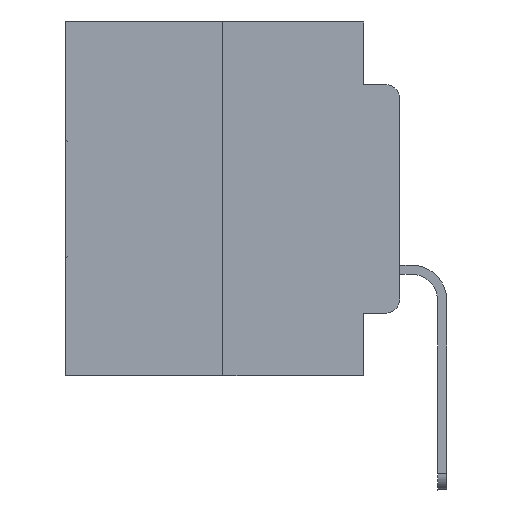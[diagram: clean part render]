
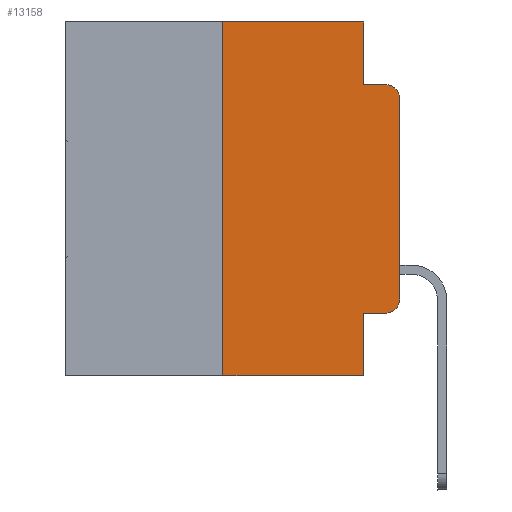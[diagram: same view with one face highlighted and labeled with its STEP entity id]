
A CAD part, left-side view. The second image highlights one B-rep face of the part: STEP entity #13158.
In plain terms, the highlighted planar face has unit normal (-1, 0, 0).
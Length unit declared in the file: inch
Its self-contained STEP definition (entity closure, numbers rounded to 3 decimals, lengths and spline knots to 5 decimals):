
#380 = LINE ( 'NONE', #9405, #19714 ) ;
#492 = DIRECTION ( 'NONE',  ( 0., 0., -1. ) ) ;
#578 = FACE_OUTER_BOUND ( 'NONE', #15499, .T. ) ;
#587 = ORIENTED_EDGE ( 'NONE', *, *, #24625, .T. ) ;
#1168 = PLANE ( 'NONE',  #5610 ) ;
#1200 = AXIS2_PLACEMENT_3D ( 'NONE', #18054, #7723, #14354 ) ;
#1474 = LINE ( 'NONE', #10653, #11525 ) ;
#1544 = CARTESIAN_POINT ( 'NONE',  ( 0., 0.02, -0.3915 ) ) ;
#1706 = VECTOR ( 'NONE', #13586, 39.37008 ) ;
#2257 = ORIENTED_EDGE ( 'NONE', *, *, #26049, .F. ) ;
#2346 = CARTESIAN_POINT ( 'NONE',  ( 0., 0.051, -0.4115 ) ) ;
#2530 = EDGE_CURVE ( 'NONE', #24203, #27634, #28332, .T. ) ;
#3697 = CIRCLE ( 'NONE', #15929, 0.02 ) ;
#4872 = CARTESIAN_POINT ( 'NONE',  ( 0., 0., 0. ) ) ;
#5607 = DIRECTION ( 'NONE',  ( 1., 0., 0. ) ) ;
#5610 = AXIS2_PLACEMENT_3D ( 'NONE', #27601, #5607, #7378 ) ;
#6230 = VERTEX_POINT ( 'NONE', #17805 ) ;
#6759 = DIRECTION ( 'NONE',  ( 0., -1., 0. ) ) ;
#7185 = DIRECTION ( 'NONE',  ( 0., 0., 1. ) ) ;
#7378 = DIRECTION ( 'NONE',  ( 0., 0., -1. ) ) ;
#7431 = CARTESIAN_POINT ( 'NONE',  ( 0., 0.051, 0. ) ) ;
#7723 = DIRECTION ( 'NONE',  ( -1., 0., 0. ) ) ;
#7748 = CARTESIAN_POINT ( 'NONE',  ( 0., 0., -0.1085 ) ) ;
#7784 = ORIENTED_EDGE ( 'NONE', *, *, #9140, .F. ) ;
#8297 = LINE ( 'NONE', #17011, #24877 ) ;
#9023 = CARTESIAN_POINT ( 'NONE',  ( 0., 0.25, 0. ) ) ;
#9140 = EDGE_CURVE ( 'NONE', #15841, #12263, #27657, .T. ) ;
#9329 = DIRECTION ( 'NONE',  ( 0., 0., -1. ) ) ;
#9405 = CARTESIAN_POINT ( 'NONE',  ( 0., 0.25, 0. ) ) ;
#10653 = CARTESIAN_POINT ( 'NONE',  ( 0., 0.051, -0.0885 ) ) ;
#10809 = ORIENTED_EDGE ( 'NONE', *, *, #21648, .T. ) ;
#11111 = CARTESIAN_POINT ( 'NONE',  ( 0., 0.051, 0. ) ) ;
#11270 = EDGE_CURVE ( 'NONE', #26734, #24547, #22586, .T. ) ;
#11525 = VECTOR ( 'NONE', #28369, 39.37008 ) ;
#11673 = VERTEX_POINT ( 'NONE', #13836 ) ;
#11846 = CARTESIAN_POINT ( 'NONE',  ( 0., 0.25, -0.5 ) ) ;
#12263 = VERTEX_POINT ( 'NONE', #21591 ) ;
#12752 = VERTEX_POINT ( 'NONE', #11846 ) ;
#13158 = ADVANCED_FACE ( 'NONE', ( #578 ), #1168, .F. ) ;
#13586 = DIRECTION ( 'NONE',  ( 0., -1., 0. ) ) ;
#13742 = CARTESIAN_POINT ( 'NONE',  ( 0., 0.473, -0.5 ) ) ;
#13836 = CARTESIAN_POINT ( 'NONE',  ( 0., 0.02, -0.0885 ) ) ;
#14354 = DIRECTION ( 'NONE',  ( 0., 0., -1. ) ) ;
#14804 = DIRECTION ( 'NONE',  ( 0., -1., 0. ) ) ;
#15499 = EDGE_LOOP ( 'NONE', ( #24904, #10809, #26312, #7784, #20578, #2257, #587, #25203, #22160, #18366 ) ) ;
#15841 = VERTEX_POINT ( 'NONE', #18964 ) ;
#15929 = AXIS2_PLACEMENT_3D ( 'NONE', #1544, #17334, #26354 ) ;
#16120 = CARTESIAN_POINT ( 'NONE',  ( 0., 0., -0.3915 ) ) ;
#16571 = VERTEX_POINT ( 'NONE', #9023 ) ;
#17011 = CARTESIAN_POINT ( 'NONE',  ( 0., 0.473, 0. ) ) ;
#17334 = DIRECTION ( 'NONE',  ( -1., 0., 0. ) ) ;
#17626 = CIRCLE ( 'NONE', #1200, 0.02 ) ;
#17805 = CARTESIAN_POINT ( 'NONE',  ( 0., 0.02, -0.4115 ) ) ;
#17972 = LINE ( 'NONE', #26983, #26885 ) ;
#18054 = CARTESIAN_POINT ( 'NONE',  ( 0., 0.02, -0.1085 ) ) ;
#18366 = ORIENTED_EDGE ( 'NONE', *, *, #26172, .T. ) ;
#18964 = CARTESIAN_POINT ( 'NONE',  ( 0., 0.051, 0. ) ) ;
#19533 = VECTOR ( 'NONE', #25260, 39.37008 ) ;
#19537 = EDGE_CURVE ( 'NONE', #26734, #6230, #17972, .T. ) ;
#19714 = VECTOR ( 'NONE', #7185, 39.37008 ) ;
#20578 = ORIENTED_EDGE ( 'NONE', *, *, #25656, .F. ) ;
#21241 = VECTOR ( 'NONE', #492, 39.37008 ) ;
#21591 = CARTESIAN_POINT ( 'NONE',  ( 0., 0.051, -0.0885 ) ) ;
#21648 = EDGE_CURVE ( 'NONE', #27634, #11673, #17626, .T. ) ;
#22160 = ORIENTED_EDGE ( 'NONE', *, *, #19537, .T. ) ;
#22452 = VECTOR ( 'NONE', #9329, 39.37008 ) ;
#22586 = LINE ( 'NONE', #11111, #22452 ) ;
#23019 = LINE ( 'NONE', #13742, #1706 ) ;
#24203 = VERTEX_POINT ( 'NONE', #16120 ) ;
#24547 = VERTEX_POINT ( 'NONE', #26590 ) ;
#24625 = EDGE_CURVE ( 'NONE', #12752, #24547, #23019, .T. ) ;
#24877 = VECTOR ( 'NONE', #14804, 39.37008 ) ;
#24904 = ORIENTED_EDGE ( 'NONE', *, *, #2530, .T. ) ;
#25203 = ORIENTED_EDGE ( 'NONE', *, *, #11270, .F. ) ;
#25260 = DIRECTION ( 'NONE',  ( 0., 0., 1. ) ) ;
#25656 = EDGE_CURVE ( 'NONE', #16571, #15841, #8297, .T. ) ;
#26049 = EDGE_CURVE ( 'NONE', #12752, #16571, #380, .T. ) ;
#26172 = EDGE_CURVE ( 'NONE', #6230, #24203, #3697, .T. ) ;
#26312 = ORIENTED_EDGE ( 'NONE', *, *, #26631, .F. ) ;
#26354 = DIRECTION ( 'NONE',  ( 0., 0., -1. ) ) ;
#26590 = CARTESIAN_POINT ( 'NONE',  ( 0., 0.051, -0.5 ) ) ;
#26631 = EDGE_CURVE ( 'NONE', #12263, #11673, #1474, .T. ) ;
#26734 = VERTEX_POINT ( 'NONE', #2346 ) ;
#26885 = VECTOR ( 'NONE', #6759, 39.37008 ) ;
#26983 = CARTESIAN_POINT ( 'NONE',  ( 0., 0.051, -0.4115 ) ) ;
#27601 = CARTESIAN_POINT ( 'NONE',  ( 0., 0.473, 0. ) ) ;
#27634 = VERTEX_POINT ( 'NONE', #7748 ) ;
#27657 = LINE ( 'NONE', #7431, #21241 ) ;
#28332 = LINE ( 'NONE', #4872, #19533 ) ;
#28369 = DIRECTION ( 'NONE',  ( 0., -1., 0. ) ) ;
